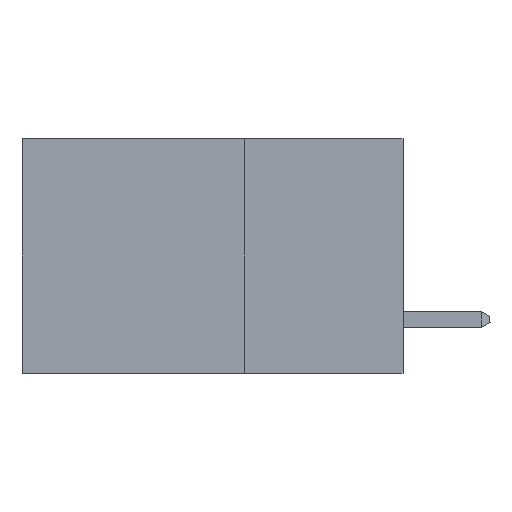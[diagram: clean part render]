
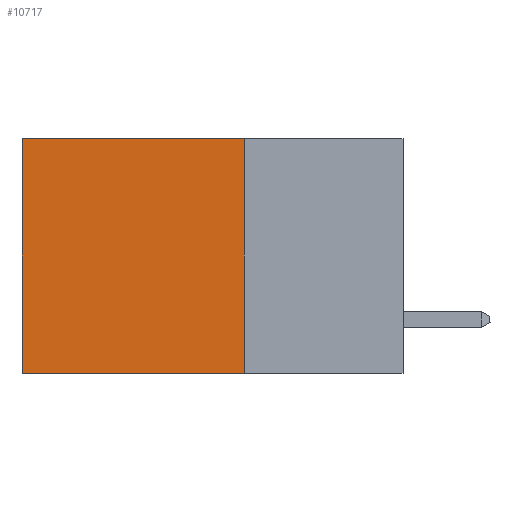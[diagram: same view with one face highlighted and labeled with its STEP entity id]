
A CAD part, left-side view. The second image highlights one B-rep face of the part: STEP entity #10717.
In plain terms, the highlighted planar face has unit normal (-1, 0, 0).
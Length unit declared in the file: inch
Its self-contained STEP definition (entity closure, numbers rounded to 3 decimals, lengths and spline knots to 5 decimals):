
#296 = FACE_OUTER_BOUND ( 'NONE', #4301, .T. ) ;
#314 = VERTEX_POINT ( 'NONE', #7691 ) ;
#561 = DIRECTION ( 'NONE',  ( 0., 0., -1. ) ) ;
#913 = VECTOR ( 'NONE', #4856, 39.37008 ) ;
#1349 = CARTESIAN_POINT ( 'NONE',  ( 0.2875, 0.25, -0.37 ) ) ;
#1505 = ORIENTED_EDGE ( 'NONE', *, *, #12094, .T. ) ;
#1768 = CARTESIAN_POINT ( 'NONE',  ( 0.2875, 0.6, 0. ) ) ;
#1771 = VERTEX_POINT ( 'NONE', #1349 ) ;
#1878 = EDGE_CURVE ( 'NONE', #1771, #314, #3777, .T. ) ;
#2276 = LINE ( 'NONE', #1768, #14666 ) ;
#2926 = EDGE_CURVE ( 'NONE', #4939, #1771, #4352, .T. ) ;
#2943 = LINE ( 'NONE', #14479, #16354 ) ;
#3089 = CARTESIAN_POINT ( 'NONE',  ( 0.2875, 0.6, 0. ) ) ;
#3777 = LINE ( 'NONE', #13417, #9438 ) ;
#3918 = DIRECTION ( 'NONE',  ( 0., 1., 0. ) ) ;
#4301 = EDGE_LOOP ( 'NONE', ( #1505, #11169, #8266, #8864 ) ) ;
#4352 = LINE ( 'NONE', #16631, #913 ) ;
#4856 = DIRECTION ( 'NONE',  ( 0., 0., -1. ) ) ;
#4939 = VERTEX_POINT ( 'NONE', #15261 ) ;
#5633 = VERTEX_POINT ( 'NONE', #3089 ) ;
#5636 = DIRECTION ( 'NONE',  ( 0., 1., 0. ) ) ;
#5816 = PLANE ( 'NONE',  #9595 ) ;
#7213 = CARTESIAN_POINT ( 'NONE',  ( 0.2875, 0.25, 0. ) ) ;
#7691 = CARTESIAN_POINT ( 'NONE',  ( 0.2875, 0.6, -0.37 ) ) ;
#8266 = ORIENTED_EDGE ( 'NONE', *, *, #2926, .F. ) ;
#8864 = ORIENTED_EDGE ( 'NONE', *, *, #9674, .T. ) ;
#9438 = VECTOR ( 'NONE', #5636, 39.37008 ) ;
#9595 = AXIS2_PLACEMENT_3D ( 'NONE', #7213, #11100, #12449 ) ;
#9674 = EDGE_CURVE ( 'NONE', #4939, #5633, #2943, .T. ) ;
#10717 = ADVANCED_FACE ( 'NONE', ( #296 ), #5816, .F. ) ;
#11100 = DIRECTION ( 'NONE',  ( 1., 0., 0. ) ) ;
#11169 = ORIENTED_EDGE ( 'NONE', *, *, #1878, .F. ) ;
#12094 = EDGE_CURVE ( 'NONE', #5633, #314, #2276, .T. ) ;
#12449 = DIRECTION ( 'NONE',  ( 0., 0., -1. ) ) ;
#13417 = CARTESIAN_POINT ( 'NONE',  ( 0.2875, 0.25, -0.37 ) ) ;
#14479 = CARTESIAN_POINT ( 'NONE',  ( 0.2875, 0.25, 0. ) ) ;
#14666 = VECTOR ( 'NONE', #561, 39.37008 ) ;
#15261 = CARTESIAN_POINT ( 'NONE',  ( 0.2875, 0.25, 0. ) ) ;
#16354 = VECTOR ( 'NONE', #3918, 39.37008 ) ;
#16631 = CARTESIAN_POINT ( 'NONE',  ( 0.2875, 0.25, 0. ) ) ;
